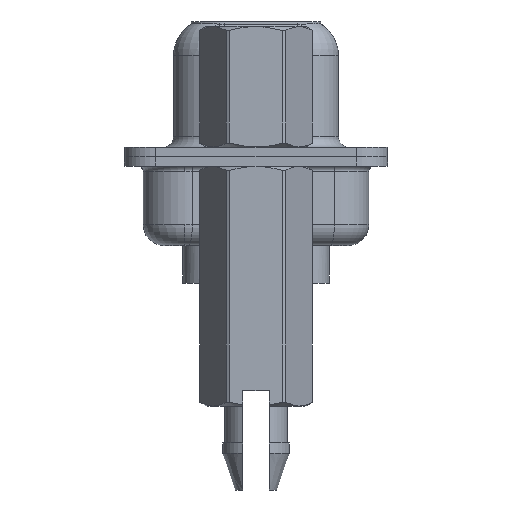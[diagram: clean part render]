
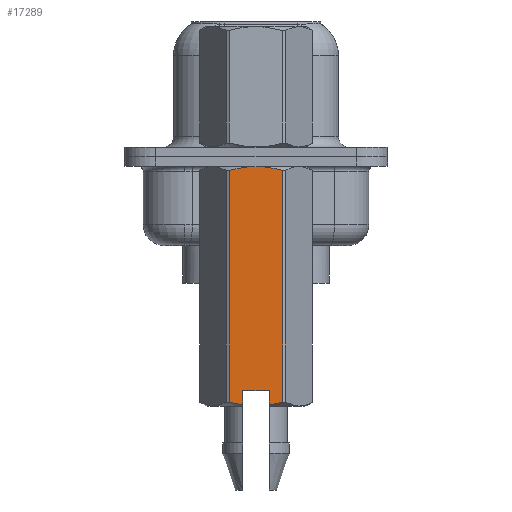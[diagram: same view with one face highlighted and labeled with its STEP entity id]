
A CAD part, left-side view. The second image highlights one B-rep face of the part: STEP entity #17289.
In plain terms, the highlighted planar face has unit normal (-1, 0, 0).
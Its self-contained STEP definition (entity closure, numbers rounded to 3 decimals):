
#735 = VERTEX_POINT ( 'NONE', #20992 ) ;
#773 = LINE ( 'NONE', #20585, #12014 ) ;
#780 = CARTESIAN_POINT ( 'NONE',  ( -2.381, -0.625, -11.885 ) ) ;
#865 = VECTOR ( 'NONE', #23244, 1000. ) ;
#1011 = EDGE_CURVE ( 'NONE', #735, #6231, #14631, .T. ) ;
#1563 = CARTESIAN_POINT ( 'NONE',  ( -2.381, -0.215, -0.468 ) ) ;
#1615 = ORIENTED_EDGE ( 'NONE', *, *, #2464, .T. ) ;
#1912 = FACE_OUTER_BOUND ( 'NONE', #5624, .T. ) ;
#1952 = VERTEX_POINT ( 'NONE', #10134 ) ;
#2464 = EDGE_CURVE ( 'NONE', #13065, #14960, #10427, .T. ) ;
#3585 = VECTOR ( 'NONE', #27346, 1000. ) ;
#3650 = PLANE ( 'NONE',  #12723 ) ;
#3826 = CARTESIAN_POINT ( 'NONE',  ( -2.381, 1.066, -0.596 ) ) ;
#3860 = CARTESIAN_POINT ( 'NONE',  ( -2.381, 0.858, -0.55 ) ) ;
#4279 = LINE ( 'NONE', #11558, #3585 ) ;
#4389 = DIRECTION ( 'NONE',  ( 0., 0., -1. ) ) ;
#5404 = CARTESIAN_POINT ( 'NONE',  ( -2.381, -1.06, -11.806 ) ) ;
#5624 = EDGE_LOOP ( 'NONE', ( #17639, #18804, #11499, #10321, #25994, #22253, #1615, #18301, #15363 ) ) ;
#5895 = DIRECTION ( 'NONE',  ( -1., 0., 0. ) ) ;
#6231 = VERTEX_POINT ( 'NONE', #18228 ) ;
#6839 = LINE ( 'NONE', #9729, #865 ) ;
#6975 = B_SPLINE_CURVE_WITH_KNOTS ( 'NONE', 3,
 ( #23078, #18490, #11785, #27576 ),
 .UNSPECIFIED., .F., .F.,
 ( 4, 4 ),
 ( 0.001, 0.002 ),
 .UNSPECIFIED. ) ;
#7302 = VERTEX_POINT ( 'NONE', #29132 ) ;
#7398 = EDGE_CURVE ( 'NONE', #7302, #1952, #4279, .T. ) ;
#7827 = EDGE_CURVE ( 'NONE', #17977, #11610, #8187, .T. ) ;
#7937 = EDGE_CURVE ( 'NONE', #14960, #20254, #773, .T. ) ;
#8187 = LINE ( 'NONE', #15576, #14148 ) ;
#8496 = CARTESIAN_POINT ( 'NONE',  ( -2.381, -0.625, -11.2 ) ) ;
#8639 = VECTOR ( 'NONE', #26304, 1000. ) ;
#8945 = CARTESIAN_POINT ( 'NONE',  ( -2.381, 1.273, -0.652 ) ) ;
#9729 = CARTESIAN_POINT ( 'NONE',  ( -2.381, -0.625, -11.2 ) ) ;
#10134 = CARTESIAN_POINT ( 'NONE',  ( -2.381, 0.625, -11.885 ) ) ;
#10321 = ORIENTED_EDGE ( 'NONE', *, *, #23444, .T. ) ;
#10427 = B_SPLINE_CURVE_WITH_KNOTS ( 'NONE', 3,
 ( #19590, #12477, #26054, #3860, #3826, #17276 ),
 .UNSPECIFIED., .F., .F.,
 ( 4, 2, 4 ),
 ( 0.004, 0.004, 0.005 ),
 .UNSPECIFIED. ) ;
#10926 = CARTESIAN_POINT ( 'NONE',  ( -2.381, 1.273, -11.748 ) ) ;
#11499 = ORIENTED_EDGE ( 'NONE', *, *, #7827, .T. ) ;
#11558 = CARTESIAN_POINT ( 'NONE',  ( -2.381, 0.625, -11.2 ) ) ;
#11610 = VERTEX_POINT ( 'NONE', #19355 ) ;
#11785 = CARTESIAN_POINT ( 'NONE',  ( -2.381, 0.845, -11.853 ) ) ;
#12014 = VECTOR ( 'NONE', #18283, 1000. ) ;
#12186 = B_SPLINE_CURVE_WITH_KNOTS ( 'NONE', 3,
 ( #780, #21059, #5404, #21152 ),
 .UNSPECIFIED., .F., .F.,
 ( 4, 4 ),
 ( 0.003, 0.004 ),
 .UNSPECIFIED. ) ;
#12477 = CARTESIAN_POINT ( 'NONE',  ( -2.381, 0.215, -0.468 ) ) ;
#12723 = AXIS2_PLACEMENT_3D ( 'NONE', #19363, #5895, #21663 ) ;
#12738 = CARTESIAN_POINT ( 'NONE',  ( -2.381, -1.065, -0.596 ) ) ;
#13065 = VERTEX_POINT ( 'NONE', #18116 ) ;
#14148 = VECTOR ( 'NONE', #4389, 1000. ) ;
#14631 = LINE ( 'NONE', #28639, #8639 ) ;
#14960 = VERTEX_POINT ( 'NONE', #8945 ) ;
#15019 = CARTESIAN_POINT ( 'NONE',  ( -2.381, -0.428, -0.485 ) ) ;
#15164 = EDGE_CURVE ( 'NONE', #17977, #7302, #6839, .T. ) ;
#15363 = ORIENTED_EDGE ( 'NONE', *, *, #20501, .T. ) ;
#15576 = CARTESIAN_POINT ( 'NONE',  ( -2.381, -0.625, -11.2 ) ) ;
#15827 = B_SPLINE_CURVE_WITH_KNOTS ( 'NONE', 3,
 ( #19447, #12738, #28513, #15019, #1563, #17270 ),
 .UNSPECIFIED., .F., .F.,
 ( 4, 2, 4 ),
 ( 0.003, 0.003, 0.004 ),
 .UNSPECIFIED. ) ;
#17270 = CARTESIAN_POINT ( 'NONE',  ( -2.381, 0., -0.468 ) ) ;
#17276 = CARTESIAN_POINT ( 'NONE',  ( -2.381, 1.273, -0.652 ) ) ;
#17289 = ADVANCED_FACE ( 'NONE', ( #1912 ), #3650, .T. ) ;
#17639 = ORIENTED_EDGE ( 'NONE', *, *, #7398, .F. ) ;
#17977 = VERTEX_POINT ( 'NONE', #8496 ) ;
#18116 = CARTESIAN_POINT ( 'NONE',  ( -2.381, 0., -0.468 ) ) ;
#18228 = CARTESIAN_POINT ( 'NONE',  ( -2.381, -1.273, -0.652 ) ) ;
#18283 = DIRECTION ( 'NONE',  ( 0., 0., -1. ) ) ;
#18301 = ORIENTED_EDGE ( 'NONE', *, *, #7937, .T. ) ;
#18490 = CARTESIAN_POINT ( 'NONE',  ( -2.381, 1.06, -11.806 ) ) ;
#18804 = ORIENTED_EDGE ( 'NONE', *, *, #15164, .F. ) ;
#19355 = CARTESIAN_POINT ( 'NONE',  ( -2.381, -0.625, -11.885 ) ) ;
#19363 = CARTESIAN_POINT ( 'NONE',  ( -2.381, -1.375, -0.45 ) ) ;
#19447 = CARTESIAN_POINT ( 'NONE',  ( -2.381, -1.273, -0.652 ) ) ;
#19590 = CARTESIAN_POINT ( 'NONE',  ( -2.381, 0., -0.468 ) ) ;
#20254 = VERTEX_POINT ( 'NONE', #10926 ) ;
#20501 = EDGE_CURVE ( 'NONE', #20254, #1952, #6975, .T. ) ;
#20585 = CARTESIAN_POINT ( 'NONE',  ( -2.381, 1.273, 0.581 ) ) ;
#20992 = CARTESIAN_POINT ( 'NONE',  ( -2.381, -1.273, -11.748 ) ) ;
#21059 = CARTESIAN_POINT ( 'NONE',  ( -2.381, -0.842, -11.854 ) ) ;
#21152 = CARTESIAN_POINT ( 'NONE',  ( -2.381, -1.273, -11.748 ) ) ;
#21663 = DIRECTION ( 'NONE',  ( 0., 0., 1. ) ) ;
#22253 = ORIENTED_EDGE ( 'NONE', *, *, #29199, .T. ) ;
#23078 = CARTESIAN_POINT ( 'NONE',  ( -2.381, 1.273, -11.748 ) ) ;
#23244 = DIRECTION ( 'NONE',  ( 0., 1., 0. ) ) ;
#23444 = EDGE_CURVE ( 'NONE', #11610, #735, #12186, .T. ) ;
#25994 = ORIENTED_EDGE ( 'NONE', *, *, #1011, .T. ) ;
#26054 = CARTESIAN_POINT ( 'NONE',  ( -2.381, 0.432, -0.485 ) ) ;
#26304 = DIRECTION ( 'NONE',  ( 0., 0., 1. ) ) ;
#27346 = DIRECTION ( 'NONE',  ( 0., 0., -1. ) ) ;
#27576 = CARTESIAN_POINT ( 'NONE',  ( -2.381, 0.625, -11.885 ) ) ;
#28513 = CARTESIAN_POINT ( 'NONE',  ( -2.381, -0.853, -0.549 ) ) ;
#28639 = CARTESIAN_POINT ( 'NONE',  ( -2.381, -1.273, 0.581 ) ) ;
#29132 = CARTESIAN_POINT ( 'NONE',  ( -2.381, 0.625, -11.2 ) ) ;
#29199 = EDGE_CURVE ( 'NONE', #6231, #13065, #15827, .T. ) ;
